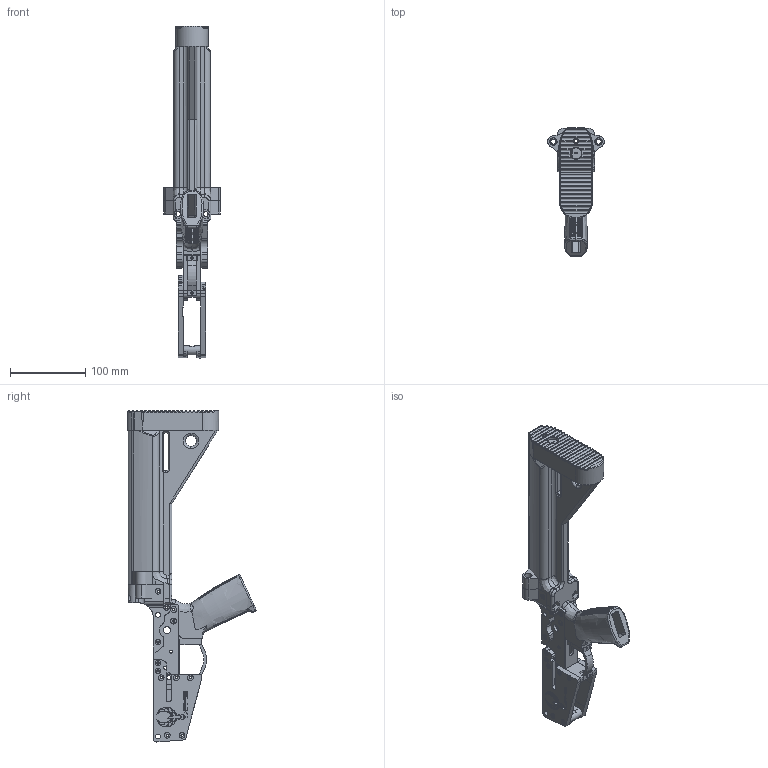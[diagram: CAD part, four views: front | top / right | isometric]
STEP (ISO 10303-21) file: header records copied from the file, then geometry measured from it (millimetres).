
FILE_DESCRIPTION (( 'STEP AP214' ), '1' );
FILE_NAME ('Firebolt_5.56_Printed_Buffer_Tube.STEP', '2020-12-05T18:50:17', ( '' ), ( '' ), 'SwSTEP 2.0', 'SolidWorks 2020', '' );
FILE_SCHEMA (( 'AUTOMOTIVE_DESIGN' ));
Length unit declared in the file: millimetre
Products named in the file (15): Firebolt_5.56_Printed_Buffer_Tube; Firebolt_Mag_Well_Right; Firebolt_Buffer_Tube; Firebolt_UBolt_Side_Left; Firebolt_Buffer_Tube_Buffer_Tower; Firebolt_UBolt_Pistol_Grip; Firebolt_UBolt_Side_Right; Firebolt_UBolt_Grip_Part; Firebolt_Buffer_Tube_Recoil_Pad; Firebolt_Trigger_Guard; Firebolt_Fire_Control_Well_Bottom; Firebolt_Mag_Well_Front; Firebolt_Mag_Well_Left; Firebolt_Mag_Well_Rear; Firebolt_Buffer_Tube_Recoil_Pad_Screw
Assembly tree (14 placements, depth 2):
  Firebolt_5.56_Printed_Buffer_Tube
    Firebolt_UBolt_Side_Left
    Firebolt_UBolt_Side_Right
    Firebolt_UBolt_Grip_Part
    Firebolt_UBolt_Pistol_Grip
    Firebolt_Fire_Control_Well_Bottom
    Firebolt_Trigger_Guard
    Firebolt_Mag_Well_Rear
    Firebolt_Mag_Well_Left
    Firebolt_Mag_Well_Front
    Firebolt_Buffer_Tube_Buffer_Tower
    Firebolt_Buffer_Tube
    Firebolt_Buffer_Tube_Recoil_Pad
    Firebolt_Mag_Well_Right
    Firebolt_Buffer_Tube_Recoil_Pad_Screw
Bounding box: 75.22 x 170.39 x 441.94 mm (x, y, z)
Volume: 771961.6 mm3; surface area: 218378.4 mm2
Topology: 14 solids, 14 shells, 2620 faces, 7819 edges, 5280 vertices
Faces by surface type: plane 1586, cylinder 663, bspline 286, torus 67, cone 11, sphere 7
Entity records: 153552 total; most frequent: CARTESIAN_POINT 81955, ORIENTED_EDGE 15630, DIRECTION 11171, EDGE_CURVE 7815, VERTEX_POINT 5280, LINE 4555, VECTOR 4555, AXIS2_PLACEMENT_3D 3308
